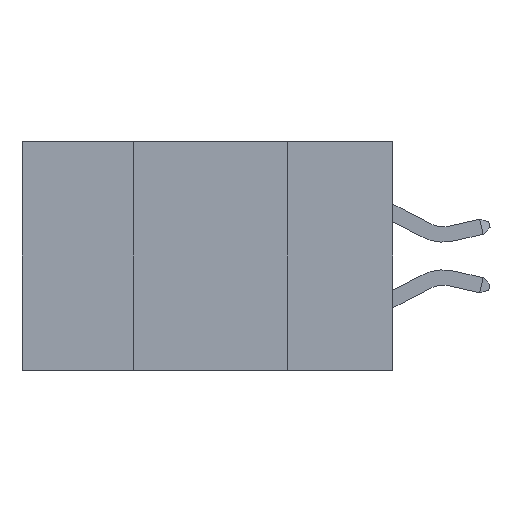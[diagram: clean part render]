
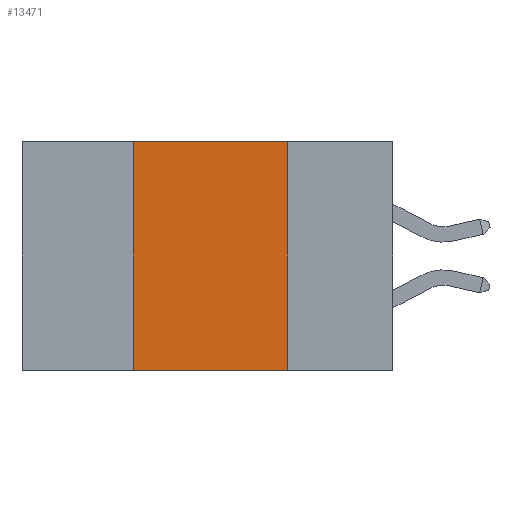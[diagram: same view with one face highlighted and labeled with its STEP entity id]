
A CAD part, left-side view. The second image highlights one B-rep face of the part: STEP entity #13471.
In plain terms, the highlighted planar face has unit normal (-1, 0, 0).
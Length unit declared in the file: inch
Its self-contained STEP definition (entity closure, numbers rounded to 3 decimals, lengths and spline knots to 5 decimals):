
#113 = CARTESIAN_POINT ( 'NONE',  ( 0., 0.17, 0. ) ) ;
#147 = AXIS2_PLACEMENT_3D ( 'NONE', #11384, #16588, #4917 ) ;
#243 = DIRECTION ( 'NONE',  ( 0., 0., 1. ) ) ;
#324 = LINE ( 'NONE', #1436, #12387 ) ;
#595 = VERTEX_POINT ( 'NONE', #7643 ) ;
#1091 = CARTESIAN_POINT ( 'NONE',  ( 0., 0.6, 0. ) ) ;
#1436 = CARTESIAN_POINT ( 'NONE',  ( 0., 0.42, 0. ) ) ;
#1700 = LINE ( 'NONE', #5614, #4157 ) ;
#2798 = CARTESIAN_POINT ( 'NONE',  ( 0., 0.42, 0. ) ) ;
#3064 = DIRECTION ( 'NONE',  ( 0., -1., 0. ) ) ;
#3411 = EDGE_CURVE ( 'NONE', #595, #8445, #10970, .T. ) ;
#3447 = EDGE_CURVE ( 'NONE', #5336, #8445, #1700, .T. ) ;
#4157 = VECTOR ( 'NONE', #6971, 39.37008 ) ;
#4514 = CARTESIAN_POINT ( 'NONE',  ( 0., 0.6, -0.37 ) ) ;
#4776 = DIRECTION ( 'NONE',  ( 0., -1., 0. ) ) ;
#4892 = ORIENTED_EDGE ( 'NONE', *, *, #14307, .F. ) ;
#4917 = DIRECTION ( 'NONE',  ( 0., 0., -1. ) ) ;
#5232 = VECTOR ( 'NONE', #3064, 39.37008 ) ;
#5336 = VERTEX_POINT ( 'NONE', #113 ) ;
#5614 = CARTESIAN_POINT ( 'NONE',  ( 0., 0.17, 0. ) ) ;
#5873 = ORIENTED_EDGE ( 'NONE', *, *, #5899, .F. ) ;
#5899 = EDGE_CURVE ( 'NONE', #595, #13151, #324, .T. ) ;
#6235 = CARTESIAN_POINT ( 'NONE',  ( 0., 0.17, -0.37 ) ) ;
#6971 = DIRECTION ( 'NONE',  ( 0., 0., -1. ) ) ;
#7394 = LINE ( 'NONE', #1091, #11862 ) ;
#7643 = CARTESIAN_POINT ( 'NONE',  ( 0., 0.42, -0.37 ) ) ;
#8445 = VERTEX_POINT ( 'NONE', #6235 ) ;
#9225 = ORIENTED_EDGE ( 'NONE', *, *, #3411, .T. ) ;
#10085 = EDGE_LOOP ( 'NONE', ( #16761, #4892, #5873, #9225 ) ) ;
#10970 = LINE ( 'NONE', #4514, #5232 ) ;
#11384 = CARTESIAN_POINT ( 'NONE',  ( 0., 0.6, 0. ) ) ;
#11862 = VECTOR ( 'NONE', #4776, 39.37008 ) ;
#12387 = VECTOR ( 'NONE', #243, 39.37008 ) ;
#13151 = VERTEX_POINT ( 'NONE', #2798 ) ;
#13471 = ADVANCED_FACE ( 'NONE', ( #14955 ), #16421, .F. ) ;
#14307 = EDGE_CURVE ( 'NONE', #13151, #5336, #7394, .T. ) ;
#14955 = FACE_OUTER_BOUND ( 'NONE', #10085, .T. ) ;
#16421 = PLANE ( 'NONE',  #147 ) ;
#16588 = DIRECTION ( 'NONE',  ( 1., 0., 0. ) ) ;
#16761 = ORIENTED_EDGE ( 'NONE', *, *, #3447, .F. ) ;
